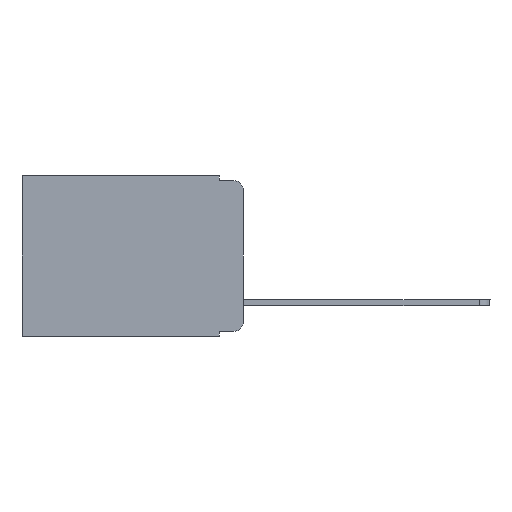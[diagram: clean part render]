
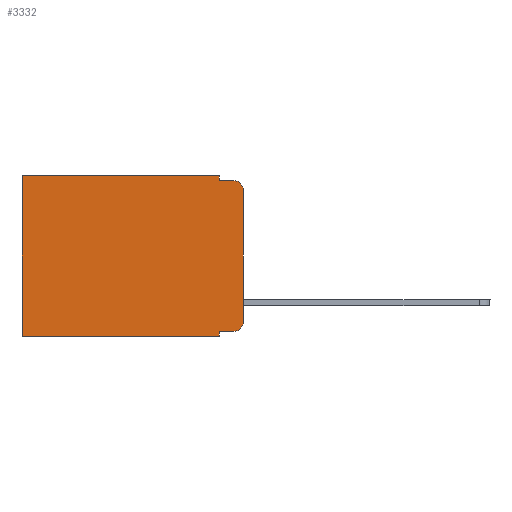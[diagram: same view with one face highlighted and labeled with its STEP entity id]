
A CAD part, left-side view. The second image highlights one B-rep face of the part: STEP entity #3332.
In plain terms, the highlighted planar face has unit normal (-1, 0, 0).
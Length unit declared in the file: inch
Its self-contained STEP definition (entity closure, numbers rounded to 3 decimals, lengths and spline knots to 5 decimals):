
#259 = ORIENTED_EDGE ( 'NONE', *, *, #12741, .T. ) ;
#582 = FACE_OUTER_BOUND ( 'NONE', #4573, .T. ) ;
#663 = EDGE_CURVE ( 'NONE', #6734, #15764, #8533, .T. ) ;
#1177 = DIRECTION ( 'NONE',  ( 0., 0., -1. ) ) ;
#1262 = VECTOR ( 'NONE', #10191, 39.37008 ) ;
#1351 = AXIS2_PLACEMENT_3D ( 'NONE', #3666, #10211, #1177 ) ;
#1695 = CARTESIAN_POINT ( 'NONE',  ( 0.298, 0.051, -0.333 ) ) ;
#1835 = EDGE_CURVE ( 'NONE', #6573, #12772, #7284, .T. ) ;
#2512 = DIRECTION ( 'NONE',  ( 0., 0., -1. ) ) ;
#2514 = VECTOR ( 'NONE', #12659, 39.37008 ) ;
#2576 = CARTESIAN_POINT ( 'NONE',  ( 0.298, 0.02, -0.313 ) ) ;
#2723 = DIRECTION ( 'NONE',  ( 0., 1., 0. ) ) ;
#3332 = ADVANCED_FACE ( 'NONE', ( #582 ), #10074, .F. ) ;
#3355 = VECTOR ( 'NONE', #2723, 39.37008 ) ;
#3459 = CIRCLE ( 'NONE', #9540, 0.02 ) ;
#3544 = CARTESIAN_POINT ( 'NONE',  ( 0.298, 0.02, -0.01 ) ) ;
#3546 = VERTEX_POINT ( 'NONE', #3544 ) ;
#3647 = DIRECTION ( 'NONE',  ( 0., 1., 0. ) ) ;
#3662 = VERTEX_POINT ( 'NONE', #10754 ) ;
#3666 = CARTESIAN_POINT ( 'NONE',  ( 0.298, 0.02, -0.03 ) ) ;
#3717 = ORIENTED_EDGE ( 'NONE', *, *, #663, .T. ) ;
#4310 = DIRECTION ( 'NONE',  ( 0., 0., -1. ) ) ;
#4385 = ORIENTED_EDGE ( 'NONE', *, *, #7325, .T. ) ;
#4493 = ORIENTED_EDGE ( 'NONE', *, *, #7473, .F. ) ;
#4573 = EDGE_LOOP ( 'NONE', ( #8736, #10786, #15611, #12007, #7780, #3717, #5727, #4493, #4385, #259 ) ) ;
#4590 = VERTEX_POINT ( 'NONE', #1695 ) ;
#5001 = CARTESIAN_POINT ( 'NONE',  ( 0.298, 0., 0. ) ) ;
#5005 = EDGE_CURVE ( 'NONE', #16509, #3546, #14186, .T. ) ;
#5099 = VERTEX_POINT ( 'NONE', #10315 ) ;
#5140 = LINE ( 'NONE', #11461, #3355 ) ;
#5324 = LINE ( 'NONE', #16616, #1262 ) ;
#5727 = ORIENTED_EDGE ( 'NONE', *, *, #10685, .F. ) ;
#6157 = EDGE_CURVE ( 'NONE', #12772, #3546, #15952, .T. ) ;
#6536 = CARTESIAN_POINT ( 'NONE',  ( 0.298, 0., 0. ) ) ;
#6573 = VERTEX_POINT ( 'NONE', #8514 ) ;
#6734 = VERTEX_POINT ( 'NONE', #10062 ) ;
#6832 = CARTESIAN_POINT ( 'NONE',  ( 0.298, 0.051, 0. ) ) ;
#6927 = VECTOR ( 'NONE', #8426, 39.37008 ) ;
#7188 = EDGE_CURVE ( 'NONE', #6573, #6734, #11927, .T. ) ;
#7284 = LINE ( 'NONE', #11118, #11292 ) ;
#7325 = EDGE_CURVE ( 'NONE', #4590, #12826, #5324, .T. ) ;
#7473 = EDGE_CURVE ( 'NONE', #4590, #3662, #12702, .T. ) ;
#7780 = ORIENTED_EDGE ( 'NONE', *, *, #7188, .T. ) ;
#7929 = DIRECTION ( 'NONE',  ( 0., 0., -1. ) ) ;
#8319 = CARTESIAN_POINT ( 'NONE',  ( 0.298, 0., -0.03 ) ) ;
#8426 = DIRECTION ( 'NONE',  ( 0., 0., -1. ) ) ;
#8514 = CARTESIAN_POINT ( 'NONE',  ( 0.298, 0.051, 0. ) ) ;
#8533 = LINE ( 'NONE', #11002, #6927 ) ;
#8736 = ORIENTED_EDGE ( 'NONE', *, *, #12859, .F. ) ;
#9540 = AXIS2_PLACEMENT_3D ( 'NONE', #2576, #11373, #2512 ) ;
#10062 = CARTESIAN_POINT ( 'NONE',  ( 0.298, 0.473, 0. ) ) ;
#10074 = PLANE ( 'NONE',  #12865 ) ;
#10191 = DIRECTION ( 'NONE',  ( 0., -1., 0. ) ) ;
#10211 = DIRECTION ( 'NONE',  ( -1., 0., 0. ) ) ;
#10315 = CARTESIAN_POINT ( 'NONE',  ( 0.298, 0., -0.313 ) ) ;
#10685 = EDGE_CURVE ( 'NONE', #3662, #15764, #5140, .T. ) ;
#10754 = CARTESIAN_POINT ( 'NONE',  ( 0.298, 0.051, -0.343 ) ) ;
#10786 = ORIENTED_EDGE ( 'NONE', *, *, #5005, .T. ) ;
#11002 = CARTESIAN_POINT ( 'NONE',  ( 0.298, 0.473, 0. ) ) ;
#11118 = CARTESIAN_POINT ( 'NONE',  ( 0.298, 0.051, 0. ) ) ;
#11230 = CARTESIAN_POINT ( 'NONE',  ( 0.298, 0.051, -0.01 ) ) ;
#11292 = VECTOR ( 'NONE', #16231, 39.37008 ) ;
#11373 = DIRECTION ( 'NONE',  ( -1., 0., 0. ) ) ;
#11376 = CARTESIAN_POINT ( 'NONE',  ( 0.298, 0., 0. ) ) ;
#11427 = DIRECTION ( 'NONE',  ( 1., 0., 0. ) ) ;
#11461 = CARTESIAN_POINT ( 'NONE',  ( 0.298, 0., -0.343 ) ) ;
#11927 = LINE ( 'NONE', #5001, #12321 ) ;
#12007 = ORIENTED_EDGE ( 'NONE', *, *, #1835, .F. ) ;
#12117 = VECTOR ( 'NONE', #4310, 39.37008 ) ;
#12321 = VECTOR ( 'NONE', #3647, 39.37008 ) ;
#12659 = DIRECTION ( 'NONE',  ( 0., -1., 0. ) ) ;
#12702 = LINE ( 'NONE', #6832, #12117 ) ;
#12710 = DIRECTION ( 'NONE',  ( 0., 0., -1. ) ) ;
#12741 = EDGE_CURVE ( 'NONE', #12826, #5099, #3459, .T. ) ;
#12772 = VERTEX_POINT ( 'NONE', #12818 ) ;
#12818 = CARTESIAN_POINT ( 'NONE',  ( 0.298, 0.051, -0.01 ) ) ;
#12826 = VERTEX_POINT ( 'NONE', #14227 ) ;
#12859 = EDGE_CURVE ( 'NONE', #16509, #5099, #14720, .T. ) ;
#12865 = AXIS2_PLACEMENT_3D ( 'NONE', #11376, #11427, #12710 ) ;
#12921 = CARTESIAN_POINT ( 'NONE',  ( 0.298, 0.473, -0.343 ) ) ;
#13067 = VECTOR ( 'NONE', #7929, 39.37008 ) ;
#14186 = CIRCLE ( 'NONE', #1351, 0.02 ) ;
#14227 = CARTESIAN_POINT ( 'NONE',  ( 0.298, 0.02, -0.333 ) ) ;
#14720 = LINE ( 'NONE', #6536, #13067 ) ;
#15611 = ORIENTED_EDGE ( 'NONE', *, *, #6157, .F. ) ;
#15764 = VERTEX_POINT ( 'NONE', #12921 ) ;
#15952 = LINE ( 'NONE', #11230, #2514 ) ;
#16231 = DIRECTION ( 'NONE',  ( 0., 0., -1. ) ) ;
#16509 = VERTEX_POINT ( 'NONE', #8319 ) ;
#16616 = CARTESIAN_POINT ( 'NONE',  ( 0.298, 0.051, -0.333 ) ) ;
